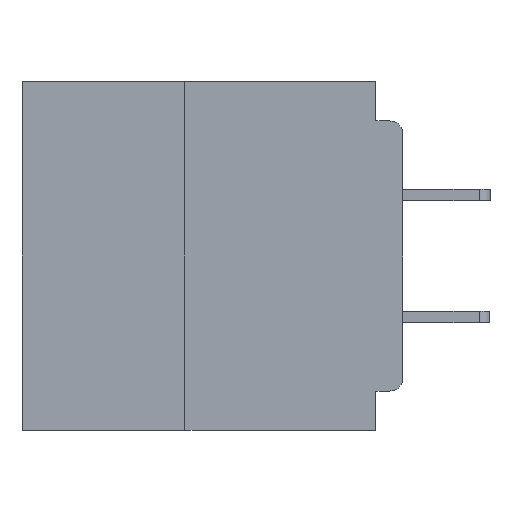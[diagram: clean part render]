
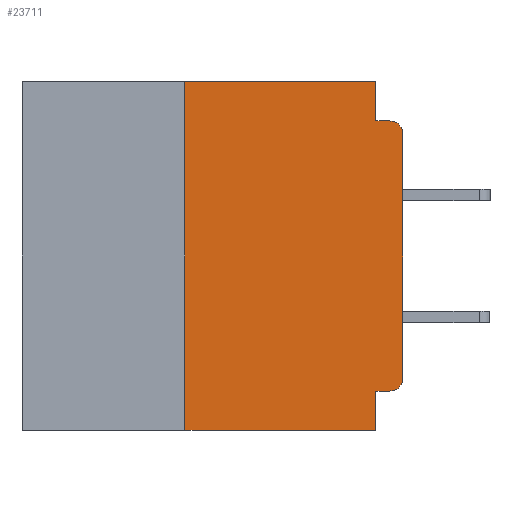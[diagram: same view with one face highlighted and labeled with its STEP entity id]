
A CAD part, left-side view. The second image highlights one B-rep face of the part: STEP entity #23711.
In plain terms, the highlighted planar face has unit normal (-1, 0, 0).
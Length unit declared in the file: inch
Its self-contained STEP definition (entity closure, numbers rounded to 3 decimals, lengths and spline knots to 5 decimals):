
#219 = VERTEX_POINT ( 'NONE', #13686 ) ;
#465 = VECTOR ( 'NONE', #33295, 39.37008 ) ;
#494 = ORIENTED_EDGE ( 'NONE', *, *, #27070, .F. ) ;
#566 = CARTESIAN_POINT ( 'NONE',  ( 0., 0.015, -0.34 ) ) ;
#1005 = VERTEX_POINT ( 'NONE', #23581 ) ;
#1081 = CARTESIAN_POINT ( 'NONE',  ( 0., 0.437, 0. ) ) ;
#2353 = DIRECTION ( 'NONE',  ( 0., 0., 1. ) ) ;
#2437 = LINE ( 'NONE', #29923, #29226 ) ;
#2571 = VECTOR ( 'NONE', #9586, 39.37008 ) ;
#2660 = DIRECTION ( 'NONE',  ( 0., 1., 0. ) ) ;
#3065 = DIRECTION ( 'NONE',  ( 0., -1., 0. ) ) ;
#3082 = CARTESIAN_POINT ( 'NONE',  ( 0., 0.031, -0.4 ) ) ;
#3169 = DIRECTION ( 'NONE',  ( 0., -1., 0. ) ) ;
#3604 = CARTESIAN_POINT ( 'NONE',  ( 0., 0.25, -0.4 ) ) ;
#3929 = DIRECTION ( 'NONE',  ( 0., 0., -1. ) ) ;
#5599 = VERTEX_POINT ( 'NONE', #22208 ) ;
#6037 = CARTESIAN_POINT ( 'NONE',  ( 0., 0., -0.355 ) ) ;
#6183 = CARTESIAN_POINT ( 'NONE',  ( 0., 0.437, -0.4 ) ) ;
#6534 = CARTESIAN_POINT ( 'NONE',  ( 0., 0.031, 0. ) ) ;
#6641 = CARTESIAN_POINT ( 'NONE',  ( 0., 0.031, -0.355 ) ) ;
#6687 = DIRECTION ( 'NONE',  ( 0., 0., -1. ) ) ;
#7269 = ORIENTED_EDGE ( 'NONE', *, *, #31717, .F. ) ;
#7864 = PLANE ( 'NONE',  #8892 ) ;
#8163 = LINE ( 'NONE', #43291, #33818 ) ;
#8425 = CIRCLE ( 'NONE', #42841, 0.015 ) ;
#8768 = ORIENTED_EDGE ( 'NONE', *, *, #24024, .F. ) ;
#8892 = AXIS2_PLACEMENT_3D ( 'NONE', #1081, #34654, #14617 ) ;
#8963 = EDGE_LOOP ( 'NONE', ( #25079, #38274, #37630, #7269, #42333, #494, #37381, #24036, #8768, #32470 ) ) ;
#9039 = VECTOR ( 'NONE', #6687, 39.37008 ) ;
#9435 = LINE ( 'NONE', #3082, #465 ) ;
#9586 = DIRECTION ( 'NONE',  ( 0., -1., 0. ) ) ;
#11557 = LINE ( 'NONE', #6183, #2571 ) ;
#12671 = VERTEX_POINT ( 'NONE', #27062 ) ;
#13686 = CARTESIAN_POINT ( 'NONE',  ( 0., 0.031, 0. ) ) ;
#13942 = LINE ( 'NONE', #31885, #38500 ) ;
#14617 = DIRECTION ( 'NONE',  ( 0., 0., -1. ) ) ;
#15582 = CARTESIAN_POINT ( 'NONE',  ( 0., 0.015, -0.06 ) ) ;
#16316 = EDGE_CURVE ( 'NONE', #30306, #36074, #8163, .T. ) ;
#17354 = FACE_OUTER_BOUND ( 'NONE', #8963, .T. ) ;
#18980 = DIRECTION ( 'NONE',  ( 0., 0., -1. ) ) ;
#19161 = EDGE_CURVE ( 'NONE', #26683, #5599, #8425, .T. ) ;
#20750 = EDGE_CURVE ( 'NONE', #28148, #36074, #34871, .T. ) ;
#22208 = CARTESIAN_POINT ( 'NONE',  ( 0., 0., -0.34 ) ) ;
#22253 = VERTEX_POINT ( 'NONE', #6641 ) ;
#22608 = LINE ( 'NONE', #6037, #39264 ) ;
#23267 = CARTESIAN_POINT ( 'NONE',  ( 0., 0.031, -0.045 ) ) ;
#23581 = CARTESIAN_POINT ( 'NONE',  ( 0., 0.25, 0. ) ) ;
#23711 = ADVANCED_FACE ( 'NONE', ( #17354 ), #7864, .F. ) ;
#24024 = EDGE_CURVE ( 'NONE', #26683, #22253, #22608, .T. ) ;
#24036 = ORIENTED_EDGE ( 'NONE', *, *, #27196, .F. ) ;
#24139 = DIRECTION ( 'NONE',  ( -1., 0., 0. ) ) ;
#25079 = ORIENTED_EDGE ( 'NONE', *, *, #36204, .T. ) ;
#25911 = CARTESIAN_POINT ( 'NONE',  ( 0., 0.25, -0.4 ) ) ;
#26683 = VERTEX_POINT ( 'NONE', #40190 ) ;
#27062 = CARTESIAN_POINT ( 'NONE',  ( 0., 0.031, -0.4 ) ) ;
#27070 = EDGE_CURVE ( 'NONE', #33455, #1005, #31463, .T. ) ;
#27133 = EDGE_CURVE ( 'NONE', #33455, #12671, #11557, .T. ) ;
#27196 = EDGE_CURVE ( 'NONE', #22253, #12671, #9435, .T. ) ;
#28148 = VERTEX_POINT ( 'NONE', #28194 ) ;
#28194 = CARTESIAN_POINT ( 'NONE',  ( 0., 0., -0.06 ) ) ;
#28485 = EDGE_CURVE ( 'NONE', #1005, #219, #2437, .T. ) ;
#28950 = LINE ( 'NONE', #6534, #9039 ) ;
#29226 = VECTOR ( 'NONE', #3065, 39.37008 ) ;
#29923 = CARTESIAN_POINT ( 'NONE',  ( 0., 0.437, 0. ) ) ;
#30306 = VERTEX_POINT ( 'NONE', #23267 ) ;
#31463 = LINE ( 'NONE', #25911, #40312 ) ;
#31717 = EDGE_CURVE ( 'NONE', #219, #30306, #28950, .T. ) ;
#31885 = CARTESIAN_POINT ( 'NONE',  ( 0., 0., 0. ) ) ;
#32470 = ORIENTED_EDGE ( 'NONE', *, *, #19161, .T. ) ;
#33295 = DIRECTION ( 'NONE',  ( 0., 0., -1. ) ) ;
#33455 = VERTEX_POINT ( 'NONE', #3604 ) ;
#33818 = VECTOR ( 'NONE', #3169, 39.37008 ) ;
#34654 = DIRECTION ( 'NONE',  ( 1., 0., 0. ) ) ;
#34871 = CIRCLE ( 'NONE', #42690, 0.015 ) ;
#35354 = DIRECTION ( 'NONE',  ( 0., 0., 1. ) ) ;
#36074 = VERTEX_POINT ( 'NONE', #41351 ) ;
#36204 = EDGE_CURVE ( 'NONE', #5599, #28148, #13942, .T. ) ;
#37381 = ORIENTED_EDGE ( 'NONE', *, *, #27133, .T. ) ;
#37630 = ORIENTED_EDGE ( 'NONE', *, *, #16316, .F. ) ;
#38274 = ORIENTED_EDGE ( 'NONE', *, *, #20750, .T. ) ;
#38500 = VECTOR ( 'NONE', #35354, 39.37008 ) ;
#38974 = DIRECTION ( 'NONE',  ( -1., 0., 0. ) ) ;
#39264 = VECTOR ( 'NONE', #2660, 39.37008 ) ;
#40190 = CARTESIAN_POINT ( 'NONE',  ( 0., 0.015, -0.355 ) ) ;
#40312 = VECTOR ( 'NONE', #2353, 39.37008 ) ;
#41351 = CARTESIAN_POINT ( 'NONE',  ( 0., 0.015, -0.045 ) ) ;
#42333 = ORIENTED_EDGE ( 'NONE', *, *, #28485, .F. ) ;
#42690 = AXIS2_PLACEMENT_3D ( 'NONE', #15582, #38974, #18980 ) ;
#42841 = AXIS2_PLACEMENT_3D ( 'NONE', #566, #24139, #3929 ) ;
#43291 = CARTESIAN_POINT ( 'NONE',  ( 0., 0., -0.045 ) ) ;
